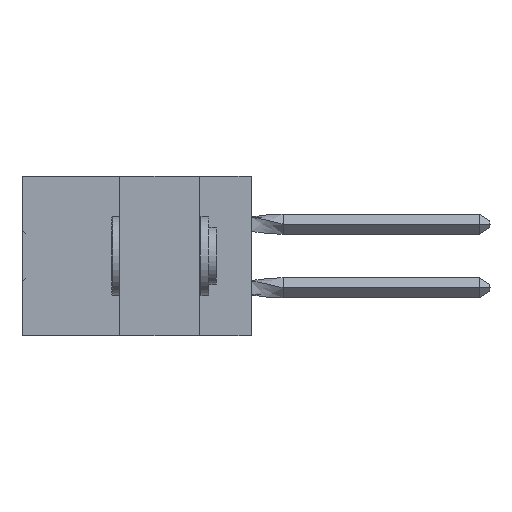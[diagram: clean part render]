
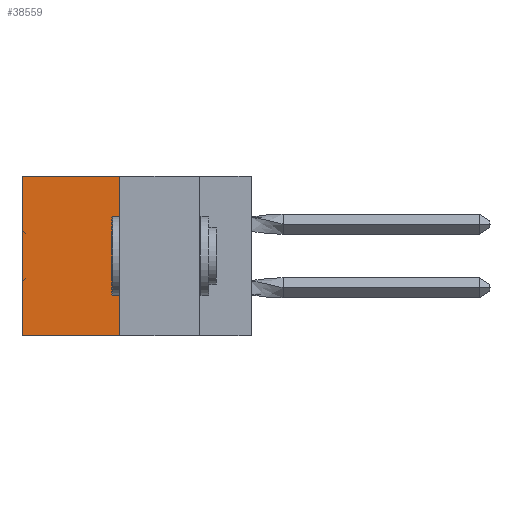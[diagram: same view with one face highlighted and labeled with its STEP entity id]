
A CAD part, left-side view. The second image highlights one B-rep face of the part: STEP entity #38559.
In plain terms, the highlighted planar face has unit normal (-1, 0, 0).
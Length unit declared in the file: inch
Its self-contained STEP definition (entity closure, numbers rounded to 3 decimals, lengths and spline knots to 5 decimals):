
#740 = LINE ( 'NONE', #4140, #43959 ) ;
#1760 = CARTESIAN_POINT ( 'NONE',  ( 0.305, 0.413, -0.5 ) ) ;
#3575 = LINE ( 'NONE', #43747, #57992 ) ;
#4140 = CARTESIAN_POINT ( 'NONE',  ( 0.305, 0.413, -0.5 ) ) ;
#4515 = EDGE_CURVE ( 'NONE', #56108, #7610, #8672, .T. ) ;
#5451 = CARTESIAN_POINT ( 'NONE',  ( 0.305, 0.72, -0.5 ) ) ;
#7610 = VERTEX_POINT ( 'NONE', #29894 ) ;
#8672 = LINE ( 'NONE', #26717, #42182 ) ;
#15108 = CARTESIAN_POINT ( 'NONE',  ( 0.305, 0.413, 0. ) ) ;
#17768 = PLANE ( 'NONE',  #57874 ) ;
#19269 = VECTOR ( 'NONE', #43009, 39.37008 ) ;
#25597 = EDGE_CURVE ( 'NONE', #7610, #44799, #56471, .T. ) ;
#26717 = CARTESIAN_POINT ( 'NONE',  ( 0.305, 0.413, 0. ) ) ;
#29894 = CARTESIAN_POINT ( 'NONE',  ( 0.305, 0.72, 0. ) ) ;
#29966 = ORIENTED_EDGE ( 'NONE', *, *, #25597, .T. ) ;
#30069 = CARTESIAN_POINT ( 'NONE',  ( 0.305, 0.72, -0.5 ) ) ;
#36034 = EDGE_CURVE ( 'NONE', #41882, #44799, #740, .T. ) ;
#36198 = ORIENTED_EDGE ( 'NONE', *, *, #36034, .F. ) ;
#37281 = DIRECTION ( 'NONE',  ( 1., 0., 0. ) ) ;
#38559 = ADVANCED_FACE ( 'NONE', ( #56263 ), #17768, .F. ) ;
#40935 = DIRECTION ( 'NONE',  ( 0., 1., 0. ) ) ;
#40989 = ORIENTED_EDGE ( 'NONE', *, *, #48908, .F. ) ;
#41882 = VERTEX_POINT ( 'NONE', #1760 ) ;
#41975 = EDGE_LOOP ( 'NONE', ( #29966, #36198, #40989, #61067 ) ) ;
#42182 = VECTOR ( 'NONE', #40935, 39.37008 ) ;
#42273 = DIRECTION ( 'NONE',  ( 0., 1., 0. ) ) ;
#43009 = DIRECTION ( 'NONE',  ( 0., 0., -1. ) ) ;
#43747 = CARTESIAN_POINT ( 'NONE',  ( 0.305, 0.413, -0.5 ) ) ;
#43959 = VECTOR ( 'NONE', #42273, 39.37008 ) ;
#44799 = VERTEX_POINT ( 'NONE', #5451 ) ;
#46753 = DIRECTION ( 'NONE',  ( 0., 0., -1. ) ) ;
#48908 = EDGE_CURVE ( 'NONE', #56108, #41882, #3575, .T. ) ;
#52660 = DIRECTION ( 'NONE',  ( 0., 0., -1. ) ) ;
#56108 = VERTEX_POINT ( 'NONE', #15108 ) ;
#56263 = FACE_OUTER_BOUND ( 'NONE', #41975, .T. ) ;
#56277 = CARTESIAN_POINT ( 'NONE',  ( 0.305, 0.413, -0.5 ) ) ;
#56471 = LINE ( 'NONE', #30069, #19269 ) ;
#57874 = AXIS2_PLACEMENT_3D ( 'NONE', #56277, #37281, #46753 ) ;
#57992 = VECTOR ( 'NONE', #52660, 39.37008 ) ;
#61067 = ORIENTED_EDGE ( 'NONE', *, *, #4515, .T. ) ;
